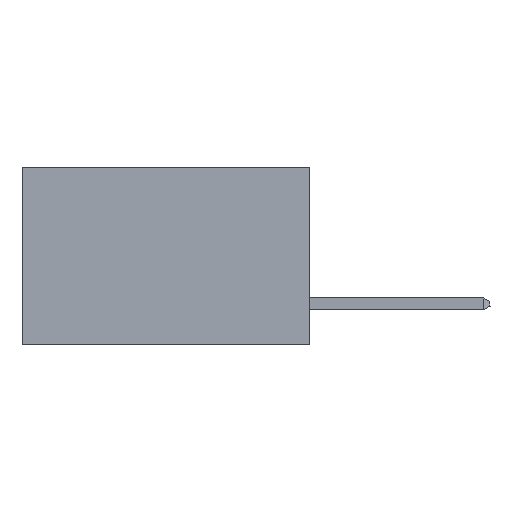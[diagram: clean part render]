
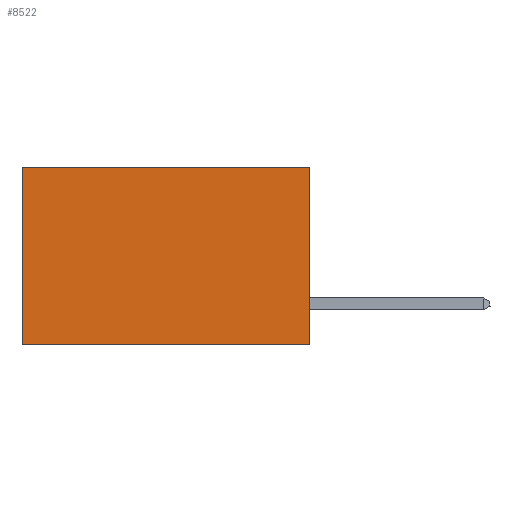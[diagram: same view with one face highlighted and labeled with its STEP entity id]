
A CAD part, left-side view. The second image highlights one B-rep face of the part: STEP entity #8522.
In plain terms, the highlighted planar face has unit normal (-1, 0, 0).
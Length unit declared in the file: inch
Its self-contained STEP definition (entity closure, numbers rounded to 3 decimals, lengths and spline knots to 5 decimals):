
#184 = DIRECTION ( 'NONE',  ( 0., 0., -1. ) ) ;
#2567 = VECTOR ( 'NONE', #31059, 39.37008 ) ;
#2899 = EDGE_CURVE ( 'NONE', #19067, #6587, #17946, .T. ) ;
#4677 = EDGE_LOOP ( 'NONE', ( #37516, #38221, #6264, #26894 ) ) ;
#5784 = EDGE_CURVE ( 'NONE', #19067, #19152, #11629, .T. ) ;
#6264 = ORIENTED_EDGE ( 'NONE', *, *, #5784, .F. ) ;
#6587 = VERTEX_POINT ( 'NONE', #41698 ) ;
#6931 = CARTESIAN_POINT ( 'NONE',  ( 0.2875, 0., -0.37 ) ) ;
#6935 = DIRECTION ( 'NONE',  ( 0., 1., 0. ) ) ;
#7990 = CARTESIAN_POINT ( 'NONE',  ( 0.2875, 0., -0.37 ) ) ;
#8522 = ADVANCED_FACE ( 'NONE', ( #33780 ), #13654, .F. ) ;
#11629 = LINE ( 'NONE', #39635, #20521 ) ;
#13489 = LINE ( 'NONE', #33422, #14591 ) ;
#13654 = PLANE ( 'NONE',  #21849 ) ;
#14591 = VECTOR ( 'NONE', #22984, 39.37008 ) ;
#15540 = LINE ( 'NONE', #6931, #2567 ) ;
#16188 = VERTEX_POINT ( 'NONE', #30937 ) ;
#17946 = LINE ( 'NONE', #27726, #38522 ) ;
#18925 = DIRECTION ( 'NONE',  ( 0., 0., -1. ) ) ;
#19067 = VERTEX_POINT ( 'NONE', #37881 ) ;
#19152 = VERTEX_POINT ( 'NONE', #7990 ) ;
#20521 = VECTOR ( 'NONE', #18925, 39.37008 ) ;
#20983 = CARTESIAN_POINT ( 'NONE',  ( 0.2875, 0., 0. ) ) ;
#21849 = AXIS2_PLACEMENT_3D ( 'NONE', #20983, #24297, #184 ) ;
#22984 = DIRECTION ( 'NONE',  ( 0., 0., -1. ) ) ;
#24297 = DIRECTION ( 'NONE',  ( 1., 0., 0. ) ) ;
#26894 = ORIENTED_EDGE ( 'NONE', *, *, #2899, .T. ) ;
#27726 = CARTESIAN_POINT ( 'NONE',  ( 0.2875, 0., 0. ) ) ;
#30165 = EDGE_CURVE ( 'NONE', #19152, #16188, #15540, .T. ) ;
#30937 = CARTESIAN_POINT ( 'NONE',  ( 0.2875, 0.6, -0.37 ) ) ;
#31059 = DIRECTION ( 'NONE',  ( 0., 1., 0. ) ) ;
#33422 = CARTESIAN_POINT ( 'NONE',  ( 0.2875, 0.6, 0. ) ) ;
#33780 = FACE_OUTER_BOUND ( 'NONE', #4677, .T. ) ;
#37516 = ORIENTED_EDGE ( 'NONE', *, *, #42665, .T. ) ;
#37881 = CARTESIAN_POINT ( 'NONE',  ( 0.2875, 0., 0. ) ) ;
#38221 = ORIENTED_EDGE ( 'NONE', *, *, #30165, .F. ) ;
#38522 = VECTOR ( 'NONE', #6935, 39.37008 ) ;
#39635 = CARTESIAN_POINT ( 'NONE',  ( 0.2875, 0., 0. ) ) ;
#41698 = CARTESIAN_POINT ( 'NONE',  ( 0.2875, 0.6, 0. ) ) ;
#42665 = EDGE_CURVE ( 'NONE', #6587, #16188, #13489, .T. ) ;
